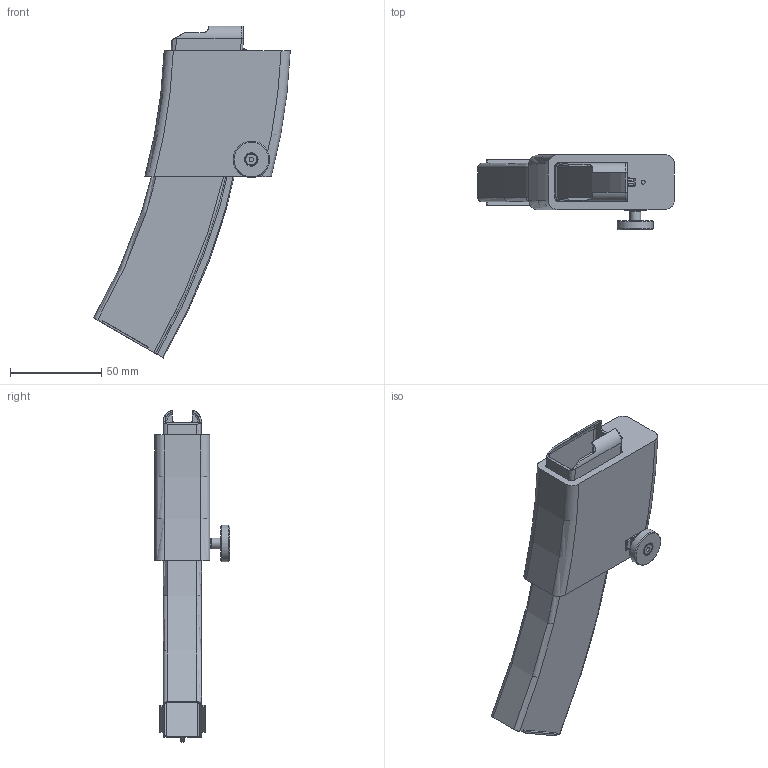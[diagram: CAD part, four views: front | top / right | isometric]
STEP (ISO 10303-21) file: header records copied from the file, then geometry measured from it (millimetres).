
FILE_DESCRIPTION(/* description */ (''),/* implementation_level */ '2;1');
FILE_NAME(/* name */ 'PPS43 Magwell .stp',/* time_stamp */ '2020-08-06T13:08:14+03:00',/* author */ (''),/* organization */ (''),/* preprocessor_version */ 'ST-DEVELOPER v15.2',/* originating_system */ 'Autodesk Translator Framework v2.0.0.5431',/* authorisation */ '');
FILE_SCHEMA (('AUTOMOTIVE_DESIGN { 1 0 10303 214 3 1 1 }'));
Length unit declared in the file: centimetre
Products named in the file (1): (Unsaved)
Bounding box: 107.58 x 41.4 x 181.71 mm (x, y, z)
Volume: 100565.1 mm3; surface area: 70045.3 mm2
Topology: 4 solids, 4 shells, 266 faces, 686 edges, 418 vertices
Faces by surface type: cylinder 87, plane 82, bspline 49, torus 33, sphere 11, cone 4
Full cylindrical faces by diameter (mm): 2.3 x1, 2.5 x2, 6 x1, 6.6 x1, 20 x1
Entity records: 10212 total; most frequent: CARTESIAN_POINT 3989, ORIENTED_EDGE 1326, DIRECTION 1253, EDGE_CURVE 663, AXIS2_PLACEMENT_3D 498, VERTEX_POINT 413, EDGE_LOOP 286, FACE_OUTER_BOUND 266
